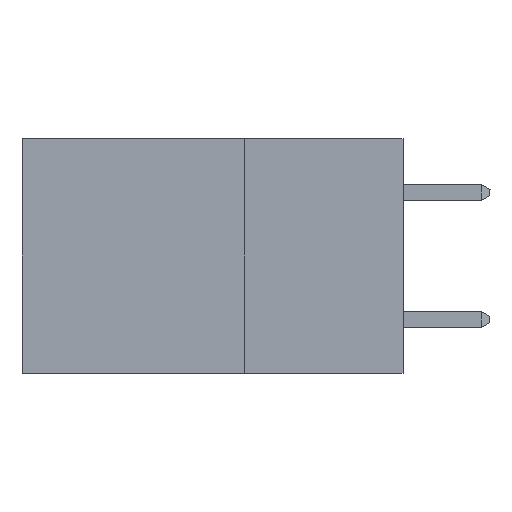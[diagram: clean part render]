
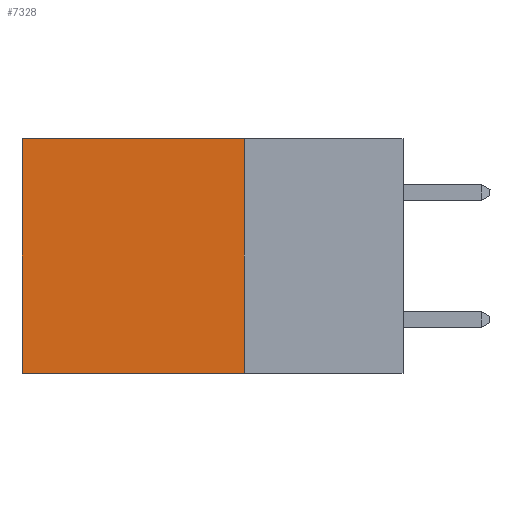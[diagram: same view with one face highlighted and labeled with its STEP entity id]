
A CAD part, left-side view. The second image highlights one B-rep face of the part: STEP entity #7328.
In plain terms, the highlighted planar face has unit normal (-1, 0, 0).
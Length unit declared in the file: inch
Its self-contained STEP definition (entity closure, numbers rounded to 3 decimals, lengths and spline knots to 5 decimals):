
#28 = DIRECTION ( 'NONE',  ( 0., 0., -1. ) ) ;
#612 = EDGE_CURVE ( 'NONE', #3390, #3117, #8412, .T. ) ;
#1791 = EDGE_CURVE ( 'NONE', #3117, #3322, #7868, .T. ) ;
#2390 = EDGE_CURVE ( 'NONE', #7287, #3322, #8203, .T. ) ;
#2996 = DIRECTION ( 'NONE',  ( 0., 1., 0. ) ) ;
#3050 = CARTESIAN_POINT ( 'NONE',  ( 0.2875, 0.6, 0. ) ) ;
#3117 = VERTEX_POINT ( 'NONE', #13377 ) ;
#3138 = CARTESIAN_POINT ( 'NONE',  ( 0.2875, 0.25, 0. ) ) ;
#3140 = DIRECTION ( 'NONE',  ( 0., 1., 0. ) ) ;
#3188 = CARTESIAN_POINT ( 'NONE',  ( 0.2875, 0.25, -0.37 ) ) ;
#3322 = VERTEX_POINT ( 'NONE', #10573 ) ;
#3390 = VERTEX_POINT ( 'NONE', #10111 ) ;
#3687 = DIRECTION ( 'NONE',  ( 0., 0., -1. ) ) ;
#5064 = VECTOR ( 'NONE', #7834, 39.37008 ) ;
#5579 = CARTESIAN_POINT ( 'NONE',  ( 0.2875, 0.25, 0. ) ) ;
#5806 = AXIS2_PLACEMENT_3D ( 'NONE', #6851, #10016, #3687 ) ;
#6171 = ORIENTED_EDGE ( 'NONE', *, *, #6951, .F. ) ;
#6851 = CARTESIAN_POINT ( 'NONE',  ( 0.2875, 0.25, 0. ) ) ;
#6951 = EDGE_CURVE ( 'NONE', #3390, #7287, #11627, .T. ) ;
#7287 = VERTEX_POINT ( 'NONE', #12005 ) ;
#7324 = ORIENTED_EDGE ( 'NONE', *, *, #1791, .T. ) ;
#7328 = ADVANCED_FACE ( 'NONE', ( #7693 ), #8971, .F. ) ;
#7693 = FACE_OUTER_BOUND ( 'NONE', #8674, .T. ) ;
#7834 = DIRECTION ( 'NONE',  ( 0., 0., -1. ) ) ;
#7868 = LINE ( 'NONE', #3050, #5064 ) ;
#8203 = LINE ( 'NONE', #3188, #11303 ) ;
#8412 = LINE ( 'NONE', #5579, #10843 ) ;
#8674 = EDGE_LOOP ( 'NONE', ( #7324, #13463, #6171, #9713 ) ) ;
#8852 = VECTOR ( 'NONE', #28, 39.37008 ) ;
#8971 = PLANE ( 'NONE',  #5806 ) ;
#9713 = ORIENTED_EDGE ( 'NONE', *, *, #612, .T. ) ;
#10016 = DIRECTION ( 'NONE',  ( 1., 0., 0. ) ) ;
#10111 = CARTESIAN_POINT ( 'NONE',  ( 0.2875, 0.25, 0. ) ) ;
#10573 = CARTESIAN_POINT ( 'NONE',  ( 0.2875, 0.6, -0.37 ) ) ;
#10843 = VECTOR ( 'NONE', #2996, 39.37008 ) ;
#11303 = VECTOR ( 'NONE', #3140, 39.37008 ) ;
#11627 = LINE ( 'NONE', #3138, #8852 ) ;
#12005 = CARTESIAN_POINT ( 'NONE',  ( 0.2875, 0.25, -0.37 ) ) ;
#13377 = CARTESIAN_POINT ( 'NONE',  ( 0.2875, 0.6, 0. ) ) ;
#13463 = ORIENTED_EDGE ( 'NONE', *, *, #2390, .F. ) ;
